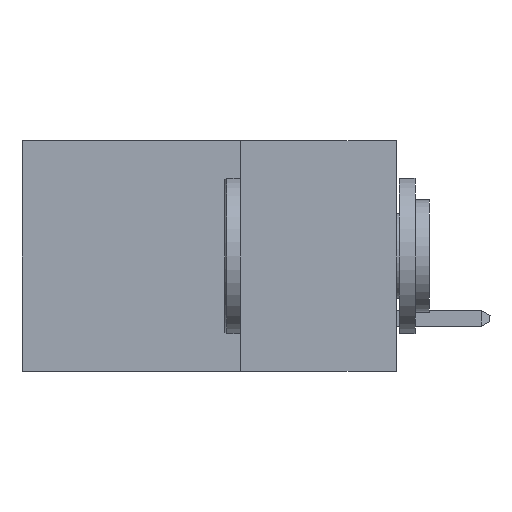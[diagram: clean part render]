
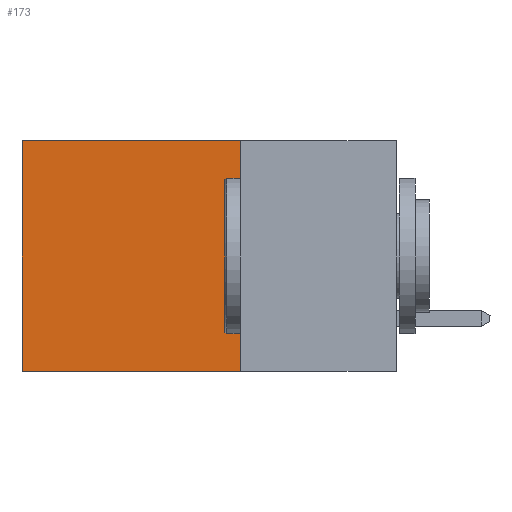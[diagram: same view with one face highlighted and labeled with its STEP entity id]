
A CAD part, left-side view. The second image highlights one B-rep face of the part: STEP entity #173.
In plain terms, the highlighted planar face has unit normal (-1, 0, 0).
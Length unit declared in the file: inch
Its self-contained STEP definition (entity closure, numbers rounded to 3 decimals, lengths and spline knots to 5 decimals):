
#119 = DIRECTION ( 'NONE',  ( 0., 1., 0. ) ) ;
#173 = ADVANCED_FACE ( 'NONE', ( #12747 ), #7537, .F. ) ;
#640 = EDGE_LOOP ( 'NONE', ( #6240, #2305, #10018, #13208 ) ) ;
#2305 = ORIENTED_EDGE ( 'NONE', *, *, #14721, .F. ) ;
#2599 = EDGE_CURVE ( 'NONE', #14214, #14025, #10579, .T. ) ;
#4924 = CARTESIAN_POINT ( 'NONE',  ( 0.2615, 0.25, 0. ) ) ;
#5143 = EDGE_CURVE ( 'NONE', #11230, #8850, #12997, .T. ) ;
#5853 = DIRECTION ( 'NONE',  ( 0., 0., -1. ) ) ;
#6240 = ORIENTED_EDGE ( 'NONE', *, *, #2599, .T. ) ;
#6403 = CARTESIAN_POINT ( 'NONE',  ( 0.2615, 0.6, -0.37 ) ) ;
#7537 = PLANE ( 'NONE',  #14560 ) ;
#7609 = CARTESIAN_POINT ( 'NONE',  ( 0.2615, 0.25, -0.37 ) ) ;
#8693 = CARTESIAN_POINT ( 'NONE',  ( 0.2615, 0.25, -0.37 ) ) ;
#8728 = DIRECTION ( 'NONE',  ( 0., 0., -1. ) ) ;
#8774 = EDGE_CURVE ( 'NONE', #11230, #14214, #14346, .T. ) ;
#8850 = VERTEX_POINT ( 'NONE', #14434 ) ;
#8867 = VECTOR ( 'NONE', #8728, 39.37008 ) ;
#9079 = LINE ( 'NONE', #7609, #11760 ) ;
#9332 = CARTESIAN_POINT ( 'NONE',  ( 0.2615, 0.25, -0.37 ) ) ;
#9492 = VECTOR ( 'NONE', #5853, 39.37008 ) ;
#10018 = ORIENTED_EDGE ( 'NONE', *, *, #5143, .F. ) ;
#10336 = DIRECTION ( 'NONE',  ( 1., 0., 0. ) ) ;
#10500 = DIRECTION ( 'NONE',  ( 0., 0., -1. ) ) ;
#10579 = LINE ( 'NONE', #6403, #9492 ) ;
#11230 = VERTEX_POINT ( 'NONE', #11940 ) ;
#11329 = VECTOR ( 'NONE', #119, 39.37008 ) ;
#11333 = CARTESIAN_POINT ( 'NONE',  ( 0.2615, 0.6, 0. ) ) ;
#11760 = VECTOR ( 'NONE', #13362, 39.37008 ) ;
#11940 = CARTESIAN_POINT ( 'NONE',  ( 0.2615, 0.25, 0. ) ) ;
#12747 = FACE_OUTER_BOUND ( 'NONE', #640, .T. ) ;
#12997 = LINE ( 'NONE', #8693, #8867 ) ;
#13208 = ORIENTED_EDGE ( 'NONE', *, *, #8774, .T. ) ;
#13362 = DIRECTION ( 'NONE',  ( 0., 1., 0. ) ) ;
#14025 = VERTEX_POINT ( 'NONE', #14368 ) ;
#14214 = VERTEX_POINT ( 'NONE', #11333 ) ;
#14346 = LINE ( 'NONE', #4924, #11329 ) ;
#14368 = CARTESIAN_POINT ( 'NONE',  ( 0.2615, 0.6, -0.37 ) ) ;
#14434 = CARTESIAN_POINT ( 'NONE',  ( 0.2615, 0.25, -0.37 ) ) ;
#14560 = AXIS2_PLACEMENT_3D ( 'NONE', #9332, #10336, #10500 ) ;
#14721 = EDGE_CURVE ( 'NONE', #8850, #14025, #9079, .T. ) ;
